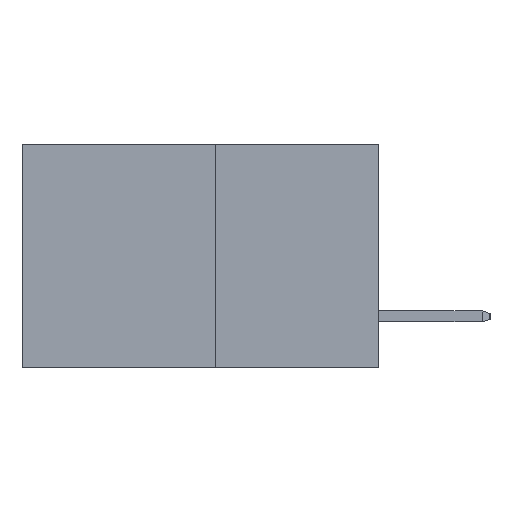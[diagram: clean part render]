
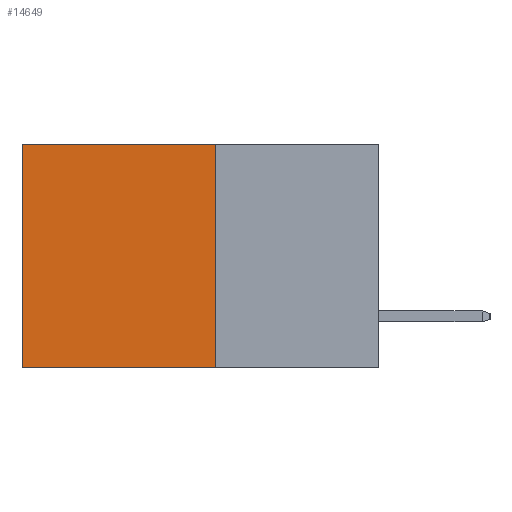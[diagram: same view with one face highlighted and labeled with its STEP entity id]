
A CAD part, left-side view. The second image highlights one B-rep face of the part: STEP entity #14649.
In plain terms, the highlighted planar face has unit normal (-1, 0, 0).
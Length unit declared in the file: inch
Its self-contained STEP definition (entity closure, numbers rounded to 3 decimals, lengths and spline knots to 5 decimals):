
#35 = FACE_OUTER_BOUND ( 'NONE', #12314, .T. ) ;
#46 = EDGE_CURVE ( 'NONE', #13329, #11340, #7528, .T. ) ;
#131 = CARTESIAN_POINT ( 'NONE',  ( 0.277, 0.59, -0.37 ) ) ;
#1186 = LINE ( 'NONE', #131, #13688 ) ;
#1356 = DIRECTION ( 'NONE',  ( 0., 1., 0. ) ) ;
#1654 = CARTESIAN_POINT ( 'NONE',  ( 0.277, 0.27, -0.37 ) ) ;
#3096 = CARTESIAN_POINT ( 'NONE',  ( 0.277, 0.27, 0. ) ) ;
#3117 = ORIENTED_EDGE ( 'NONE', *, *, #10334, .F. ) ;
#3222 = ORIENTED_EDGE ( 'NONE', *, *, #46, .T. ) ;
#4903 = CARTESIAN_POINT ( 'NONE',  ( 0.277, 0.59, 0. ) ) ;
#5030 = DIRECTION ( 'NONE',  ( 1., 0., 0. ) ) ;
#5271 = VERTEX_POINT ( 'NONE', #12967 ) ;
#5822 = AXIS2_PLACEMENT_3D ( 'NONE', #10941, #5030, #13333 ) ;
#6084 = EDGE_CURVE ( 'NONE', #11340, #5271, #1186, .T. ) ;
#6147 = LINE ( 'NONE', #15268, #8916 ) ;
#6433 = DIRECTION ( 'NONE',  ( 0., 0., -1. ) ) ;
#7145 = VECTOR ( 'NONE', #1356, 39.37008 ) ;
#7528 = LINE ( 'NONE', #3096, #7145 ) ;
#8279 = VECTOR ( 'NONE', #12570, 39.37008 ) ;
#8916 = VECTOR ( 'NONE', #10572, 39.37008 ) ;
#9177 = CARTESIAN_POINT ( 'NONE',  ( 0.277, 0.27, 0. ) ) ;
#9710 = PLANE ( 'NONE',  #5822 ) ;
#10334 = EDGE_CURVE ( 'NONE', #13329, #12769, #15000, .T. ) ;
#10572 = DIRECTION ( 'NONE',  ( 0., 1., 0. ) ) ;
#10941 = CARTESIAN_POINT ( 'NONE',  ( 0.277, 0.27, -0.37 ) ) ;
#11340 = VERTEX_POINT ( 'NONE', #4903 ) ;
#11542 = ORIENTED_EDGE ( 'NONE', *, *, #6084, .T. ) ;
#12314 = EDGE_LOOP ( 'NONE', ( #11542, #14281, #3117, #3222 ) ) ;
#12570 = DIRECTION ( 'NONE',  ( 0., 0., -1. ) ) ;
#12769 = VERTEX_POINT ( 'NONE', #14215 ) ;
#12967 = CARTESIAN_POINT ( 'NONE',  ( 0.277, 0.59, -0.37 ) ) ;
#13329 = VERTEX_POINT ( 'NONE', #9177 ) ;
#13333 = DIRECTION ( 'NONE',  ( 0., 0., -1. ) ) ;
#13688 = VECTOR ( 'NONE', #6433, 39.37008 ) ;
#14215 = CARTESIAN_POINT ( 'NONE',  ( 0.277, 0.27, -0.37 ) ) ;
#14281 = ORIENTED_EDGE ( 'NONE', *, *, #14450, .F. ) ;
#14450 = EDGE_CURVE ( 'NONE', #12769, #5271, #6147, .T. ) ;
#14649 = ADVANCED_FACE ( 'NONE', ( #35 ), #9710, .F. ) ;
#15000 = LINE ( 'NONE', #1654, #8279 ) ;
#15268 = CARTESIAN_POINT ( 'NONE',  ( 0.277, 0.27, -0.37 ) ) ;
